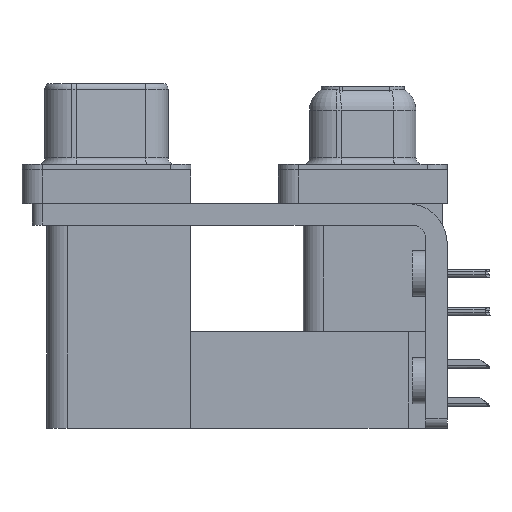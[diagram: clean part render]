
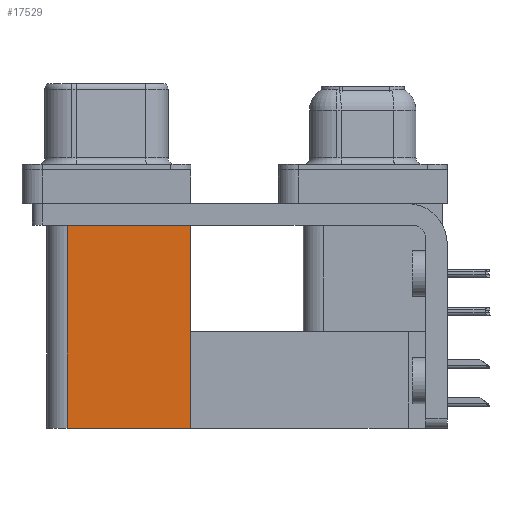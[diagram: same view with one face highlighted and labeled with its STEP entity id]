
A CAD part, left-side view. The second image highlights one B-rep face of the part: STEP entity #17529.
In plain terms, the highlighted planar face has unit normal (-1, 0, 0).
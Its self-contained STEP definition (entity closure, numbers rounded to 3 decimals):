
#183 = VERTEX_POINT ( 'NONE', #21295 ) ;
#809 = VERTEX_POINT ( 'NONE', #43769 ) ;
#904 = CARTESIAN_POINT ( 'NONE',  ( 3.765, 21.975, -2.5 ) ) ;
#1692 = PLANE ( 'NONE',  #21896 ) ;
#2889 = CARTESIAN_POINT ( 'NONE',  ( 3.765, 12.775, -19.2 ) ) ;
#4510 = LINE ( 'NONE', #18099, #21406 ) ;
#5194 = EDGE_LOOP ( 'NONE', ( #16768, #37769, #7425, #23876 ) ) ;
#7007 = CARTESIAN_POINT ( 'NONE',  ( 3.765, 12.775, -19.2 ) ) ;
#7425 = ORIENTED_EDGE ( 'NONE', *, *, #26727, .F. ) ;
#7838 = CARTESIAN_POINT ( 'NONE',  ( 3.765, 21.975, -19.2 ) ) ;
#10340 = LINE ( 'NONE', #7007, #30529 ) ;
#11160 = VECTOR ( 'NONE', #43307, 1000. ) ;
#14100 = EDGE_CURVE ( 'NONE', #809, #22198, #35939, .T. ) ;
#16768 = ORIENTED_EDGE ( 'NONE', *, *, #14100, .T. ) ;
#17529 = ADVANCED_FACE ( 'NONE', ( #32203 ), #1692, .F. ) ;
#18015 = EDGE_CURVE ( 'NONE', #183, #22198, #21439, .T. ) ;
#18099 = CARTESIAN_POINT ( 'NONE',  ( 3.765, 12.775, -19.2 ) ) ;
#18640 = DIRECTION ( 'NONE',  ( 0., 0., -1. ) ) ;
#20874 = EDGE_CURVE ( 'NONE', #39068, #809, #4510, .T. ) ;
#21295 = CARTESIAN_POINT ( 'NONE',  ( 3.765, 21.975, -19.2 ) ) ;
#21406 = VECTOR ( 'NONE', #31663, 1000. ) ;
#21439 = LINE ( 'NONE', #7838, #25475 ) ;
#21646 = DIRECTION ( 'NONE',  ( 0., 0., 1. ) ) ;
#21896 = AXIS2_PLACEMENT_3D ( 'NONE', #22643, #32423, #18640 ) ;
#22198 = VERTEX_POINT ( 'NONE', #904 ) ;
#22643 = CARTESIAN_POINT ( 'NONE',  ( 3.765, 12.775, -19.2 ) ) ;
#23876 = ORIENTED_EDGE ( 'NONE', *, *, #20874, .T. ) ;
#25475 = VECTOR ( 'NONE', #21646, 1000. ) ;
#26727 = EDGE_CURVE ( 'NONE', #39068, #183, #10340, .T. ) ;
#29715 = CARTESIAN_POINT ( 'NONE',  ( 3.765, 12.775, -2.5 ) ) ;
#30529 = VECTOR ( 'NONE', #34593, 1000. ) ;
#31663 = DIRECTION ( 'NONE',  ( 0., 0., 1. ) ) ;
#32203 = FACE_OUTER_BOUND ( 'NONE', #5194, .T. ) ;
#32423 = DIRECTION ( 'NONE',  ( 1., 0., 0. ) ) ;
#34593 = DIRECTION ( 'NONE',  ( 0., 1., 0. ) ) ;
#35939 = LINE ( 'NONE', #29715, #11160 ) ;
#37769 = ORIENTED_EDGE ( 'NONE', *, *, #18015, .F. ) ;
#39068 = VERTEX_POINT ( 'NONE', #2889 ) ;
#43307 = DIRECTION ( 'NONE',  ( 0., 1., 0. ) ) ;
#43769 = CARTESIAN_POINT ( 'NONE',  ( 3.765, 12.775, -2.5 ) ) ;
